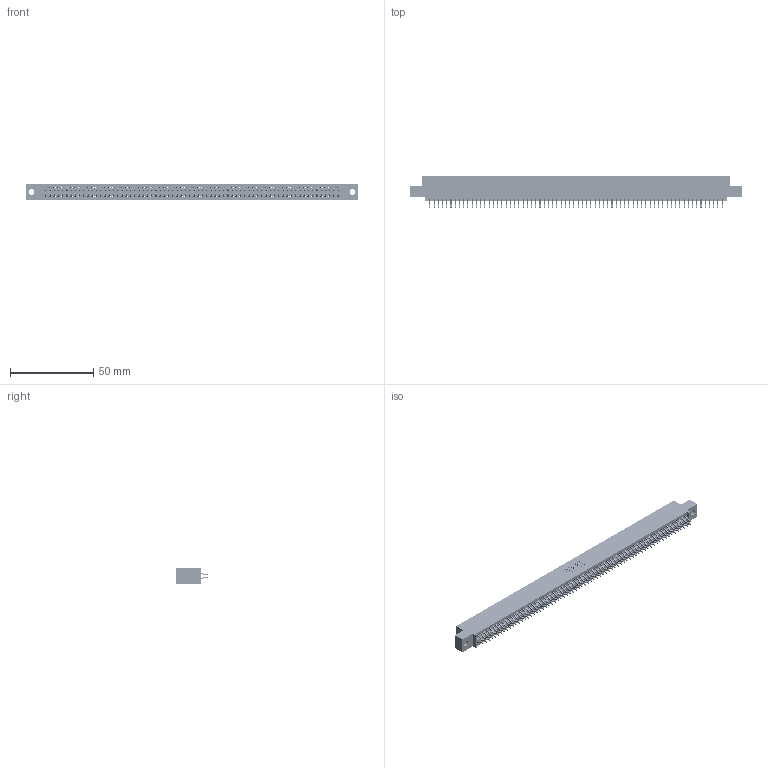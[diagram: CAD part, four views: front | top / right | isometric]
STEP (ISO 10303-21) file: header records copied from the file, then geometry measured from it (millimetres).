
FILE_DESCRIPTION (( 'STEP AP203' ), '1' );
FILE_NAME ('345-140-556-502.STEP', '2019-11-08T22:41:08', ( '' ), ( '' ), 'SwSTEP 2.0', 'SolidWorks 2016', '' );
FILE_SCHEMA (( 'CONFIG_CONTROL_DESIGN' ));
Length unit declared in the file: inch
Products named in the file (3): 345-292-001_556 Tail; 345 Part_0.110 Offset - 0.128 Dia; 345-140-556-502
Assembly tree (141 placements, depth 2):
  345-140-556-502
    345 Part_0.110 Offset - 0.128 Dia
    345-292-001_556 Tail  x140
Bounding box: 199.01 x 19.24 x 9.4 mm (x, y, z)
Volume: 19476.3 mm3; surface area: 29029 mm2
Topology: 141 solids, 141 shells, 7970 faces, 23733 edges, 15634 vertices
Faces by surface type: plane 5264, cylinder 2706
Entity records: 51509 total; most frequent: CARTESIAN_POINT 8624, ORIENTED_EDGE 8546, DIRECTION 7557, EDGE_CURVE 4273, LINE 3853, VECTOR 3853, VERTEX_POINT 2846, AXIS2_PLACEMENT_3D 1852
